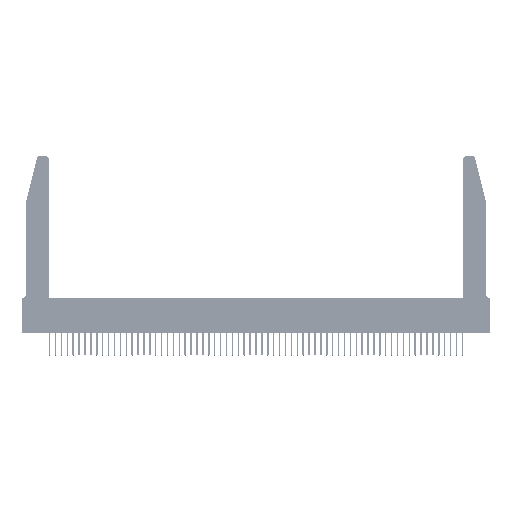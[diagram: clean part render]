
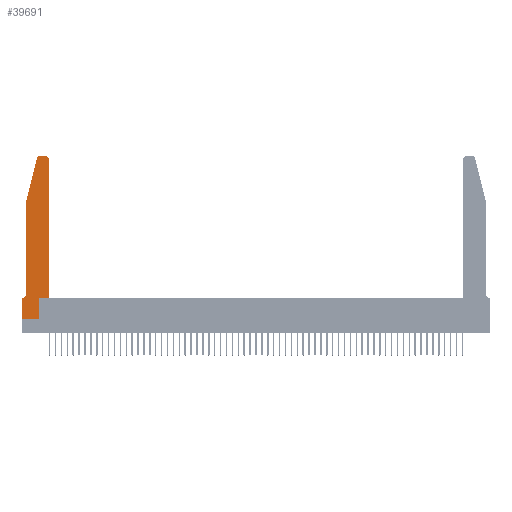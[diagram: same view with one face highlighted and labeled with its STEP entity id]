
A CAD part, top view. The second image highlights one B-rep face of the part: STEP entity #39691.
In plain terms, the highlighted planar face has unit normal (0, 0, 1).
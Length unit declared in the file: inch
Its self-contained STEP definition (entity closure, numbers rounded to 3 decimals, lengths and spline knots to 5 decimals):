
#210 = EDGE_CURVE ( 'NONE', #14585, #32912, #4904, .T. ) ;
#318 = CARTESIAN_POINT ( 'NONE',  ( 0.25487, 2.72718, 0.37 ) ) ;
#609 = DIRECTION ( 'NONE',  ( 0., -1., 0. ) ) ;
#980 = DIRECTION ( 'NONE',  ( 0., 0., -1. ) ) ;
#1145 = DIRECTION ( 'NONE',  ( 0., 0., 1. ) ) ;
#1178 = CARTESIAN_POINT ( 'NONE',  ( 0.0055, 0.42, 0.37 ) ) ;
#2055 = DIRECTION ( 'NONE',  ( 1., 0., 0. ) ) ;
#2108 = CIRCLE ( 'NONE', #45492, 0.07 ) ;
#2137 = VERTEX_POINT ( 'NONE', #10635 ) ;
#2161 = CARTESIAN_POINT ( 'NONE',  ( 0.0755, 2., 0.37 ) ) ;
#2718 = CARTESIAN_POINT ( 'NONE',  ( 0.0755, 2., 0.37 ) ) ;
#2851 = LINE ( 'NONE', #21675, #6248 ) ;
#2890 = ORIENTED_EDGE ( 'NONE', *, *, #35554, .T. ) ;
#3443 = VERTEX_POINT ( 'NONE', #43186 ) ;
#4904 = LINE ( 'NONE', #38798, #6910 ) ;
#5467 = VECTOR ( 'NONE', #56214, 39.37008 ) ;
#6059 = LINE ( 'NONE', #2718, #14224 ) ;
#6208 = VERTEX_POINT ( 'NONE', #21974 ) ;
#6248 = VECTOR ( 'NONE', #27012, 39.37008 ) ;
#6910 = VECTOR ( 'NONE', #29427, 39.37008 ) ;
#6961 = CARTESIAN_POINT ( 'NONE',  ( 0.284, 2.75, 0.37 ) ) ;
#8372 = EDGE_CURVE ( 'NONE', #32912, #3443, #32914, .T. ) ;
#9531 = VERTEX_POINT ( 'NONE', #6961 ) ;
#9561 = ORIENTED_EDGE ( 'NONE', *, *, #44737, .T. ) ;
#10413 = VERTEX_POINT ( 'NONE', #33586 ) ;
#10635 = CARTESIAN_POINT ( 'NONE',  ( 0., 0.35, 0.37 ) ) ;
#11078 = VERTEX_POINT ( 'NONE', #46908 ) ;
#13190 = EDGE_LOOP ( 'NONE', ( #15690, #18962, #48863, #19294, #53378, #32219, #9561, #26228, #44650, #14541, #23787, #2890 ) ) ;
#13771 = PLANE ( 'NONE',  #51457 ) ;
#14224 = VECTOR ( 'NONE', #24610, 39.37008 ) ;
#14541 = ORIENTED_EDGE ( 'NONE', *, *, #210, .T. ) ;
#14585 = VERTEX_POINT ( 'NONE', #21065 ) ;
#15071 = CARTESIAN_POINT ( 'NONE',  ( 0.4205, 2.75, 0.37 ) ) ;
#15579 = EDGE_CURVE ( 'NONE', #28446, #6208, #44701, .T. ) ;
#15690 = ORIENTED_EDGE ( 'NONE', *, *, #18002, .T. ) ;
#17316 = LINE ( 'NONE', #46767, #39202 ) ;
#17568 = VECTOR ( 'NONE', #609, 39.37008 ) ;
#18002 = EDGE_CURVE ( 'NONE', #47310, #9531, #2851, .T. ) ;
#18526 = DIRECTION ( 'NONE',  ( 1., 0., 0. ) ) ;
#18533 = VECTOR ( 'NONE', #34582, 39.37008 ) ;
#18757 = EDGE_CURVE ( 'NONE', #9531, #56377, #36912, .T. ) ;
#18938 = LINE ( 'NONE', #26783, #17568 ) ;
#18962 = ORIENTED_EDGE ( 'NONE', *, *, #18757, .T. ) ;
#19071 = DIRECTION ( 'NONE',  ( 1., 0., 0. ) ) ;
#19294 = ORIENTED_EDGE ( 'NONE', *, *, #49343, .T. ) ;
#19459 = CIRCLE ( 'NONE', #52473, 0.03 ) ;
#19794 = CARTESIAN_POINT ( 'NONE',  ( 0., 0., 0.37 ) ) ;
#21065 = CARTESIAN_POINT ( 'NONE',  ( 0.2865, 0.35, 0.37 ) ) ;
#21675 = CARTESIAN_POINT ( 'NONE',  ( 0.2605, 2.75, 0.37 ) ) ;
#21974 = CARTESIAN_POINT ( 'NONE',  ( 0.2865, 0., 0.37 ) ) ;
#22101 = EDGE_CURVE ( 'NONE', #11078, #2137, #17316, .T. ) ;
#23614 = CARTESIAN_POINT ( 'NONE',  ( 0.4505, 0.35, 0.37 ) ) ;
#23623 = CARTESIAN_POINT ( 'NONE',  ( 0.284, 2.72, 0.37 ) ) ;
#23787 = ORIENTED_EDGE ( 'NONE', *, *, #8372, .T. ) ;
#24143 = VECTOR ( 'NONE', #2055, 39.37008 ) ;
#24380 = EDGE_CURVE ( 'NONE', #10413, #11078, #2108, .T. ) ;
#24610 = DIRECTION ( 'NONE',  ( 0., -1., 0. ) ) ;
#24947 = DIRECTION ( 'NONE',  ( -1., 0., 0. ) ) ;
#26228 = ORIENTED_EDGE ( 'NONE', *, *, #15579, .T. ) ;
#26783 = CARTESIAN_POINT ( 'NONE',  ( 0., 0., 0.37 ) ) ;
#27012 = DIRECTION ( 'NONE',  ( -1., 0., 0. ) ) ;
#27305 = LINE ( 'NONE', #47653, #5467 ) ;
#27769 = EDGE_CURVE ( 'NONE', #56377, #50247, #46600, .T. ) ;
#28118 = VECTOR ( 'NONE', #32704, 39.37008 ) ;
#28446 = VERTEX_POINT ( 'NONE', #51098 ) ;
#29427 = DIRECTION ( 'NONE',  ( 1., 0., 0. ) ) ;
#32219 = ORIENTED_EDGE ( 'NONE', *, *, #22101, .T. ) ;
#32704 = DIRECTION ( 'NONE',  ( -0.239, -0.971, 0. ) ) ;
#32912 = VERTEX_POINT ( 'NONE', #23614 ) ;
#32914 = LINE ( 'NONE', #47585, #18533 ) ;
#33586 = CARTESIAN_POINT ( 'NONE',  ( 0.0755, 0.42, 0.37 ) ) ;
#34123 = DIRECTION ( 'NONE',  ( 1., 0., 0. ) ) ;
#34582 = DIRECTION ( 'NONE',  ( 0., 1., 0. ) ) ;
#35554 = EDGE_CURVE ( 'NONE', #3443, #47310, #19459, .T. ) ;
#36912 = CIRCLE ( 'NONE', #51169, 0.03 ) ;
#38328 = DIRECTION ( 'NONE',  ( 0., 0., 1. ) ) ;
#38798 = CARTESIAN_POINT ( 'NONE',  ( 0.4505, 0.35, 0.37 ) ) ;
#39202 = VECTOR ( 'NONE', #24947, 39.37008 ) ;
#39691 = ADVANCED_FACE ( 'NONE', ( #47981 ), #13771, .T. ) ;
#40320 = CARTESIAN_POINT ( 'NONE',  ( 0., 0.35, 0.37 ) ) ;
#41826 = EDGE_CURVE ( 'NONE', #6208, #14585, #27305, .T. ) ;
#42735 = CARTESIAN_POINT ( 'NONE',  ( 0.4205, 2.72, 0.37 ) ) ;
#43186 = CARTESIAN_POINT ( 'NONE',  ( 0.4505, 2.72, 0.37 ) ) ;
#44650 = ORIENTED_EDGE ( 'NONE', *, *, #41826, .T. ) ;
#44701 = LINE ( 'NONE', #19794, #24143 ) ;
#44733 = DIRECTION ( 'NONE',  ( 0., 0., 1. ) ) ;
#44737 = EDGE_CURVE ( 'NONE', #2137, #28446, #18938, .T. ) ;
#45492 = AXIS2_PLACEMENT_3D ( 'NONE', #1178, #980, #50479 ) ;
#46600 = LINE ( 'NONE', #2161, #28118 ) ;
#46767 = CARTESIAN_POINT ( 'NONE',  ( 0.0755, 0.35, 0.37 ) ) ;
#46908 = CARTESIAN_POINT ( 'NONE',  ( 0.0055, 0.35, 0.37 ) ) ;
#47310 = VERTEX_POINT ( 'NONE', #15071 ) ;
#47585 = CARTESIAN_POINT ( 'NONE',  ( 0.4505, 0.35, 0.37 ) ) ;
#47653 = CARTESIAN_POINT ( 'NONE',  ( 0.2865, 0.35, 0.37 ) ) ;
#47981 = FACE_OUTER_BOUND ( 'NONE', #13190, .T. ) ;
#48863 = ORIENTED_EDGE ( 'NONE', *, *, #27769, .T. ) ;
#49343 = EDGE_CURVE ( 'NONE', #50247, #10413, #6059, .T. ) ;
#49754 = CARTESIAN_POINT ( 'NONE',  ( 0.0755, 2., 0.37 ) ) ;
#50247 = VERTEX_POINT ( 'NONE', #49754 ) ;
#50479 = DIRECTION ( 'NONE',  ( -1., 0., 0. ) ) ;
#51098 = CARTESIAN_POINT ( 'NONE',  ( 0., 0., 0.37 ) ) ;
#51169 = AXIS2_PLACEMENT_3D ( 'NONE', #23623, #1145, #19071 ) ;
#51457 = AXIS2_PLACEMENT_3D ( 'NONE', #40320, #44733, #18526 ) ;
#52473 = AXIS2_PLACEMENT_3D ( 'NONE', #42735, #38328, #34123 ) ;
#53378 = ORIENTED_EDGE ( 'NONE', *, *, #24380, .T. ) ;
#56214 = DIRECTION ( 'NONE',  ( 0., 1., 0. ) ) ;
#56377 = VERTEX_POINT ( 'NONE', #318 ) ;
